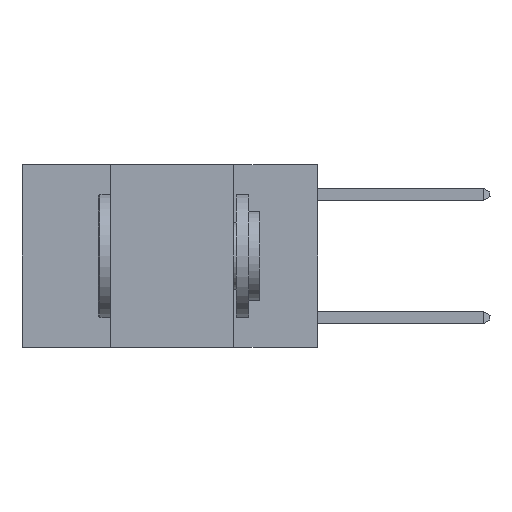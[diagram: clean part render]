
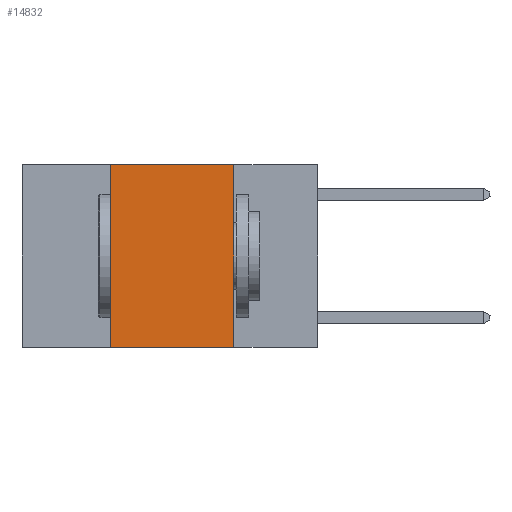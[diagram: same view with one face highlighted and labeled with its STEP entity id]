
A CAD part, left-side view. The second image highlights one B-rep face of the part: STEP entity #14832.
In plain terms, the highlighted planar face has unit normal (-1, 0, 0).
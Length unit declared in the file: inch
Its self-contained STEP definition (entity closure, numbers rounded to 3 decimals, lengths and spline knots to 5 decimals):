
#664 = DIRECTION ( 'NONE',  ( 0., 0., 1. ) ) ;
#919 = FACE_OUTER_BOUND ( 'NONE', #13159, .T. ) ;
#1563 = CARTESIAN_POINT ( 'NONE',  ( 0., 0.17, 0. ) ) ;
#2448 = LINE ( 'NONE', #11082, #4131 ) ;
#2831 = ORIENTED_EDGE ( 'NONE', *, *, #14923, .F. ) ;
#3864 = LINE ( 'NONE', #6435, #4548 ) ;
#3925 = DIRECTION ( 'NONE',  ( 0., -1., 0. ) ) ;
#4131 = VECTOR ( 'NONE', #7168, 39.37008 ) ;
#4411 = VECTOR ( 'NONE', #664, 39.37008 ) ;
#4548 = VECTOR ( 'NONE', #12285, 39.37008 ) ;
#4774 = VERTEX_POINT ( 'NONE', #1563 ) ;
#5165 = VECTOR ( 'NONE', #3925, 39.37008 ) ;
#5702 = VERTEX_POINT ( 'NONE', #11743 ) ;
#5833 = ORIENTED_EDGE ( 'NONE', *, *, #6854, .T. ) ;
#6435 = CARTESIAN_POINT ( 'NONE',  ( 0., 0.6, -0.37 ) ) ;
#6785 = DIRECTION ( 'NONE',  ( 1., 0., 0. ) ) ;
#6854 = EDGE_CURVE ( 'NONE', #7887, #14357, #3864, .T. ) ;
#6882 = AXIS2_PLACEMENT_3D ( 'NONE', #13894, #6785, #14979 ) ;
#7014 = PLANE ( 'NONE',  #6882 ) ;
#7168 = DIRECTION ( 'NONE',  ( 0., 0., -1. ) ) ;
#7285 = ORIENTED_EDGE ( 'NONE', *, *, #13294, .F. ) ;
#7887 = VERTEX_POINT ( 'NONE', #9718 ) ;
#8826 = CARTESIAN_POINT ( 'NONE',  ( 0., 0.42, 0. ) ) ;
#9718 = CARTESIAN_POINT ( 'NONE',  ( 0., 0.42, -0.37 ) ) ;
#10176 = LINE ( 'NONE', #8826, #4411 ) ;
#10966 = LINE ( 'NONE', #14439, #5165 ) ;
#11082 = CARTESIAN_POINT ( 'NONE',  ( 0., 0.17, 0. ) ) ;
#11137 = CARTESIAN_POINT ( 'NONE',  ( 0., 0.17, -0.37 ) ) ;
#11743 = CARTESIAN_POINT ( 'NONE',  ( 0., 0.42, 0. ) ) ;
#11771 = ORIENTED_EDGE ( 'NONE', *, *, #13687, .F. ) ;
#12285 = DIRECTION ( 'NONE',  ( 0., -1., 0. ) ) ;
#13159 = EDGE_LOOP ( 'NONE', ( #11771, #7285, #2831, #5833 ) ) ;
#13294 = EDGE_CURVE ( 'NONE', #5702, #4774, #10966, .T. ) ;
#13687 = EDGE_CURVE ( 'NONE', #4774, #14357, #2448, .T. ) ;
#13894 = CARTESIAN_POINT ( 'NONE',  ( 0., 0.6, 0. ) ) ;
#14357 = VERTEX_POINT ( 'NONE', #11137 ) ;
#14439 = CARTESIAN_POINT ( 'NONE',  ( 0., 0.6, 0. ) ) ;
#14832 = ADVANCED_FACE ( 'NONE', ( #919 ), #7014, .F. ) ;
#14923 = EDGE_CURVE ( 'NONE', #7887, #5702, #10176, .T. ) ;
#14979 = DIRECTION ( 'NONE',  ( 0., 0., -1. ) ) ;
